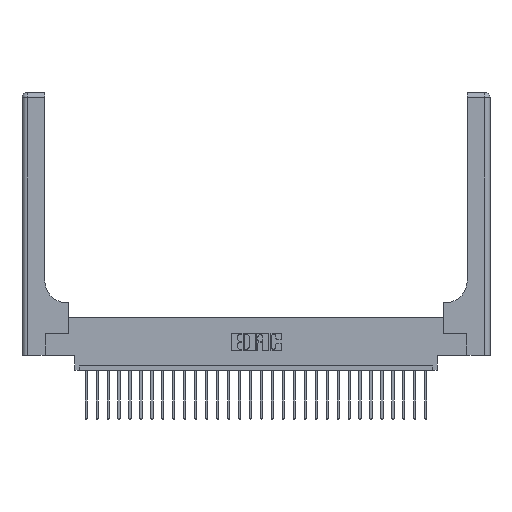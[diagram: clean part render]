
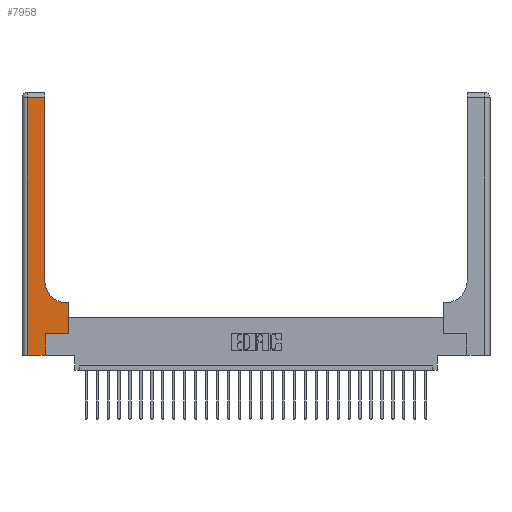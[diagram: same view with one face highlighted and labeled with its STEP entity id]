
A CAD part, top view. The second image highlights one B-rep face of the part: STEP entity #7958.
In plain terms, the highlighted planar face has unit normal (0, 0, 1).
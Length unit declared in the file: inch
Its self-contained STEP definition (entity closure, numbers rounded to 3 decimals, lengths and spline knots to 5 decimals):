
#569 = CARTESIAN_POINT ( 'NONE',  ( 0.51, 0.6, 0.37 ) ) ;
#753 = ORIENTED_EDGE ( 'NONE', *, *, #10529, .T. ) ;
#1233 = VERTEX_POINT ( 'NONE', #6414 ) ;
#1234 = CARTESIAN_POINT ( 'NONE',  ( 0., 3., 0.37 ) ) ;
#1762 = LINE ( 'NONE', #11514, #8489 ) ;
#2167 = CARTESIAN_POINT ( 'NONE',  ( 0.528, 0.6, 0.37 ) ) ;
#2183 = EDGE_CURVE ( 'NONE', #1233, #18905, #23412, .T. ) ;
#3215 = DIRECTION ( 'NONE',  ( -1., 0., 0. ) ) ;
#3847 = ORIENTED_EDGE ( 'NONE', *, *, #14239, .T. ) ;
#4709 = CARTESIAN_POINT ( 'NONE',  ( 0., 0., 0.37 ) ) ;
#4716 = ORIENTED_EDGE ( 'NONE', *, *, #21713, .T. ) ;
#4848 = VECTOR ( 'NONE', #5068, 39.37008 ) ;
#5068 = DIRECTION ( 'NONE',  ( 0., 1., 0. ) ) ;
#5085 = CARTESIAN_POINT ( 'NONE',  ( 0.265, 0.25, 0.37 ) ) ;
#5431 = CARTESIAN_POINT ( 'NONE',  ( 0.06, 0., 0.37 ) ) ;
#5432 = AXIS2_PLACEMENT_3D ( 'NONE', #24944, #16554, #12449 ) ;
#5794 = VECTOR ( 'NONE', #10819, 39.37008 ) ;
#6414 = CARTESIAN_POINT ( 'NONE',  ( 0.528, 0.25, 0.37 ) ) ;
#7132 = VECTOR ( 'NONE', #23770, 39.37008 ) ;
#7335 = VERTEX_POINT ( 'NONE', #569 ) ;
#7958 = ADVANCED_FACE ( 'NONE', ( #10588 ), #9430, .F. ) ;
#8200 = CARTESIAN_POINT ( 'NONE',  ( 0.06, 2.94, 0.37 ) ) ;
#8234 = LINE ( 'NONE', #25791, #16277 ) ;
#8344 = VERTEX_POINT ( 'NONE', #10397 ) ;
#8489 = VECTOR ( 'NONE', #11769, 39.37008 ) ;
#8613 = LINE ( 'NONE', #16551, #24640 ) ;
#8893 = DIRECTION ( 'NONE',  ( 1., 0., 0. ) ) ;
#9095 = DIRECTION ( 'NONE',  ( 0., 0., -1. ) ) ;
#9430 = PLANE ( 'NONE',  #21992 ) ;
#9633 = CIRCLE ( 'NONE', #5432, 0.25 ) ;
#9795 = ORIENTED_EDGE ( 'NONE', *, *, #2183, .T. ) ;
#10339 = CARTESIAN_POINT ( 'NONE',  ( 0.26, 0.85, 0.37 ) ) ;
#10397 = CARTESIAN_POINT ( 'NONE',  ( 0.26, 2.94, 0.37 ) ) ;
#10529 = EDGE_CURVE ( 'NONE', #18905, #7335, #8234, .T. ) ;
#10588 = FACE_OUTER_BOUND ( 'NONE', #25048, .T. ) ;
#10599 = VERTEX_POINT ( 'NONE', #8200 ) ;
#10819 = DIRECTION ( 'NONE',  ( 0., 1., 0. ) ) ;
#11514 = CARTESIAN_POINT ( 'NONE',  ( 0.265, 0., 0.37 ) ) ;
#11769 = DIRECTION ( 'NONE',  ( 0., 1., 0. ) ) ;
#11782 = EDGE_CURVE ( 'NONE', #14456, #23917, #1762, .T. ) ;
#11970 = VERTEX_POINT ( 'NONE', #10339 ) ;
#12328 = DIRECTION ( 'NONE',  ( -1., 0., 0. ) ) ;
#12449 = DIRECTION ( 'NONE',  ( 1., 0., 0. ) ) ;
#12885 = EDGE_CURVE ( 'NONE', #11970, #8344, #15757, .T. ) ;
#13081 = CARTESIAN_POINT ( 'NONE',  ( 0.26, 3., 0.37 ) ) ;
#13359 = DIRECTION ( 'NONE',  ( 0., -1., 0. ) ) ;
#13628 = EDGE_CURVE ( 'NONE', #20365, #14456, #24078, .T. ) ;
#13723 = LINE ( 'NONE', #23310, #20828 ) ;
#13771 = EDGE_CURVE ( 'NONE', #23917, #1233, #22776, .T. ) ;
#14239 = EDGE_CURVE ( 'NONE', #8344, #10599, #8613, .T. ) ;
#14456 = VERTEX_POINT ( 'NONE', #14624 ) ;
#14624 = CARTESIAN_POINT ( 'NONE',  ( 0.265, 0., 0.37 ) ) ;
#15743 = ORIENTED_EDGE ( 'NONE', *, *, #11782, .T. ) ;
#15757 = LINE ( 'NONE', #13081, #4848 ) ;
#16174 = ORIENTED_EDGE ( 'NONE', *, *, #19261, .T. ) ;
#16277 = VECTOR ( 'NONE', #26037, 39.37008 ) ;
#16432 = CARTESIAN_POINT ( 'NONE',  ( 0.265, 0.25, 0.37 ) ) ;
#16551 = CARTESIAN_POINT ( 'NONE',  ( 0., 2.94, 0.37 ) ) ;
#16554 = DIRECTION ( 'NONE',  ( 0., 0., -1. ) ) ;
#16831 = ORIENTED_EDGE ( 'NONE', *, *, #12885, .T. ) ;
#16959 = ORIENTED_EDGE ( 'NONE', *, *, #13771, .T. ) ;
#18905 = VERTEX_POINT ( 'NONE', #2167 ) ;
#19261 = EDGE_CURVE ( 'NONE', #7335, #11970, #9633, .T. ) ;
#19377 = ORIENTED_EDGE ( 'NONE', *, *, #13628, .T. ) ;
#20365 = VERTEX_POINT ( 'NONE', #5431 ) ;
#20828 = VECTOR ( 'NONE', #13359, 39.37008 ) ;
#21713 = EDGE_CURVE ( 'NONE', #10599, #20365, #13723, .T. ) ;
#21992 = AXIS2_PLACEMENT_3D ( 'NONE', #1234, #9095, #3215 ) ;
#22662 = CARTESIAN_POINT ( 'NONE',  ( 0.528, 0.25, 0.37 ) ) ;
#22776 = LINE ( 'NONE', #5085, #7132 ) ;
#23310 = CARTESIAN_POINT ( 'NONE',  ( 0.06, 3., 0.37 ) ) ;
#23412 = LINE ( 'NONE', #22662, #5794 ) ;
#23770 = DIRECTION ( 'NONE',  ( 1., 0., 0. ) ) ;
#23917 = VERTEX_POINT ( 'NONE', #16432 ) ;
#24078 = LINE ( 'NONE', #4709, #24733 ) ;
#24640 = VECTOR ( 'NONE', #12328, 39.37008 ) ;
#24733 = VECTOR ( 'NONE', #8893, 39.37008 ) ;
#24944 = CARTESIAN_POINT ( 'NONE',  ( 0.51, 0.85, 0.37 ) ) ;
#25048 = EDGE_LOOP ( 'NONE', ( #16831, #3847, #4716, #19377, #15743, #16959, #9795, #753, #16174 ) ) ;
#25791 = CARTESIAN_POINT ( 'NONE',  ( 0.26, 0.6, 0.37 ) ) ;
#26037 = DIRECTION ( 'NONE',  ( -1., 0., 0. ) ) ;
